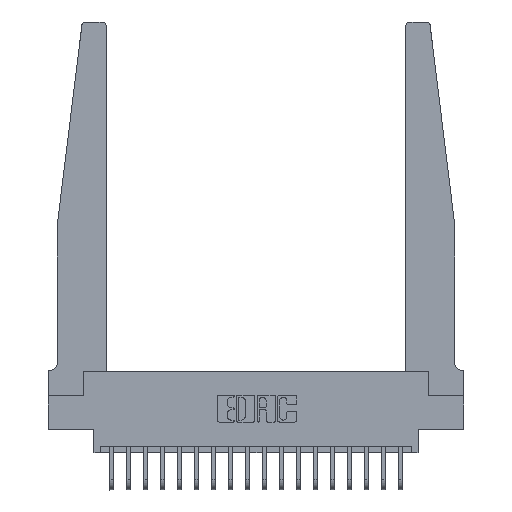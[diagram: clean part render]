
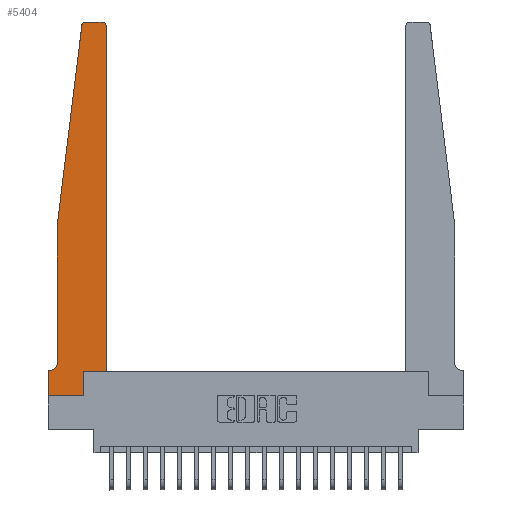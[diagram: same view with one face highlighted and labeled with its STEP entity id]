
A CAD part, top view. The second image highlights one B-rep face of the part: STEP entity #5404.
In plain terms, the highlighted planar face has unit normal (0, 0, 1).
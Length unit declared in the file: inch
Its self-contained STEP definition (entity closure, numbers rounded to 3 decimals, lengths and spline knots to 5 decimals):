
#7 = DIRECTION ( 'NONE',  ( 0., 0., -1. ) ) ;
#114 = DIRECTION ( 'NONE',  ( 1., 0., 0. ) ) ;
#468 = CARTESIAN_POINT ( 'NONE',  ( 0.24675, 2.72367, 0.37 ) ) ;
#535 = EDGE_CURVE ( 'NONE', #9507, #10295, #10881, .T. ) ;
#549 = VERTEX_POINT ( 'NONE', #468 ) ;
#550 = CIRCLE ( 'NONE', #14992, 0.03 ) ;
#697 = VERTEX_POINT ( 'NONE', #18527 ) ;
#717 = DIRECTION ( 'NONE',  ( 0., -1., 0. ) ) ;
#861 = DIRECTION ( 'NONE',  ( 0., 0., 1. ) ) ;
#1441 = CARTESIAN_POINT ( 'NONE',  ( 0., 0., 0.37 ) ) ;
#1549 = VECTOR ( 'NONE', #114, 39.37008 ) ;
#1551 = FACE_OUTER_BOUND ( 'NONE', #19303, .T. ) ;
#1722 = LINE ( 'NONE', #13590, #2767 ) ;
#2453 = CARTESIAN_POINT ( 'NONE',  ( 0.425, 0.18, 0.37 ) ) ;
#2677 = CARTESIAN_POINT ( 'NONE',  ( 0.2605, 0.18, 0.37 ) ) ;
#2767 = VECTOR ( 'NONE', #7425, 39.37008 ) ;
#2812 = VERTEX_POINT ( 'NONE', #18369 ) ;
#2819 = ORIENTED_EDGE ( 'NONE', *, *, #2838, .T. ) ;
#2838 = EDGE_CURVE ( 'NONE', #14471, #10114, #16302, .T. ) ;
#3021 = CARTESIAN_POINT ( 'NONE',  ( 0.065, 1.25, 0.37 ) ) ;
#3446 = DIRECTION ( 'NONE',  ( 0., 0., 1. ) ) ;
#3517 = ORIENTED_EDGE ( 'NONE', *, *, #6738, .T. ) ;
#3747 = CARTESIAN_POINT ( 'NONE',  ( 0.425, 0.18, 0.37 ) ) ;
#4168 = CARTESIAN_POINT ( 'NONE',  ( 0.425, 2.72, 0.37 ) ) ;
#4404 = ORIENTED_EDGE ( 'NONE', *, *, #9298, .T. ) ;
#5031 = DIRECTION ( 'NONE',  ( -1., 0., 0. ) ) ;
#5090 = CARTESIAN_POINT ( 'NONE',  ( 0.2605, 0., 0.37 ) ) ;
#5404 = ADVANCED_FACE ( 'NONE', ( #1551 ), #14762, .T. ) ;
#5718 = ORIENTED_EDGE ( 'NONE', *, *, #12366, .T. ) ;
#6118 = CIRCLE ( 'NONE', #12478, 0.03 ) ;
#6351 = EDGE_CURVE ( 'NONE', #10114, #13738, #1722, .T. ) ;
#6361 = DIRECTION ( 'NONE',  ( 1., 0., 0. ) ) ;
#6429 = EDGE_CURVE ( 'NONE', #12772, #21199, #9536, .T. ) ;
#6506 = CARTESIAN_POINT ( 'NONE',  ( 0., 0.1875, 0.37 ) ) ;
#6641 = LINE ( 'NONE', #11664, #10573 ) ;
#6738 = EDGE_CURVE ( 'NONE', #549, #10972, #9307, .T. ) ;
#6746 = ORIENTED_EDGE ( 'NONE', *, *, #6429, .T. ) ;
#6799 = VECTOR ( 'NONE', #16878, 39.37008 ) ;
#6945 = DIRECTION ( 'NONE',  ( -0.122, -0.992, 0. ) ) ;
#7122 = ORIENTED_EDGE ( 'NONE', *, *, #16498, .T. ) ;
#7391 = AXIS2_PLACEMENT_3D ( 'NONE', #20221, #7, #20282 ) ;
#7425 = DIRECTION ( 'NONE',  ( -1., 0., 0. ) ) ;
#7553 = DIRECTION ( 'NONE',  ( 0., 1., 0. ) ) ;
#7672 = EDGE_CURVE ( 'NONE', #10295, #2812, #6118, .T. ) ;
#7897 = EDGE_CURVE ( 'NONE', #2812, #697, #6641, .T. ) ;
#8036 = ORIENTED_EDGE ( 'NONE', *, *, #535, .T. ) ;
#9072 = CARTESIAN_POINT ( 'NONE',  ( 0., 0., 0.37 ) ) ;
#9298 = EDGE_CURVE ( 'NONE', #697, #549, #550, .T. ) ;
#9307 = LINE ( 'NONE', #17565, #16384 ) ;
#9326 = VECTOR ( 'NONE', #21129, 39.37008 ) ;
#9507 = VERTEX_POINT ( 'NONE', #3747 ) ;
#9510 = CARTESIAN_POINT ( 'NONE',  ( 0., 0.1875, 0.37 ) ) ;
#9536 = LINE ( 'NONE', #2677, #9326 ) ;
#9836 = VECTOR ( 'NONE', #16049, 39.37008 ) ;
#10013 = CARTESIAN_POINT ( 'NONE',  ( 0.2605, 0.18, 0.37 ) ) ;
#10114 = VERTEX_POINT ( 'NONE', #18724 ) ;
#10295 = VERTEX_POINT ( 'NONE', #4168 ) ;
#10573 = VECTOR ( 'NONE', #5031, 39.37008 ) ;
#10617 = VECTOR ( 'NONE', #7553, 39.37008 ) ;
#10620 = DIRECTION ( 'NONE',  ( 1., 0., 0. ) ) ;
#10634 = EDGE_CURVE ( 'NONE', #10870, #12772, #17252, .T. ) ;
#10870 = VERTEX_POINT ( 'NONE', #14080 ) ;
#10881 = LINE ( 'NONE', #16935, #10617 ) ;
#10972 = VERTEX_POINT ( 'NONE', #3021 ) ;
#11229 = LINE ( 'NONE', #18343, #6799 ) ;
#11637 = LINE ( 'NONE', #2453, #9836 ) ;
#11664 = CARTESIAN_POINT ( 'NONE',  ( 0.25, 2.75, 0.37 ) ) ;
#12366 = EDGE_CURVE ( 'NONE', #13738, #10870, #19293, .T. ) ;
#12478 = AXIS2_PLACEMENT_3D ( 'NONE', #13370, #3446, #10620 ) ;
#12591 = ORIENTED_EDGE ( 'NONE', *, *, #7672, .T. ) ;
#12772 = VERTEX_POINT ( 'NONE', #5090 ) ;
#12907 = ORIENTED_EDGE ( 'NONE', *, *, #7897, .T. ) ;
#13370 = CARTESIAN_POINT ( 'NONE',  ( 0.395, 2.72, 0.37 ) ) ;
#13590 = CARTESIAN_POINT ( 'NONE',  ( 0.065, 0.1875, 0.37 ) ) ;
#13738 = VERTEX_POINT ( 'NONE', #9510 ) ;
#14080 = CARTESIAN_POINT ( 'NONE',  ( 0., 0., 0.37 ) ) ;
#14471 = VERTEX_POINT ( 'NONE', #16854 ) ;
#14659 = EDGE_CURVE ( 'NONE', #10972, #14471, #11229, .T. ) ;
#14762 = PLANE ( 'NONE',  #21441 ) ;
#14992 = AXIS2_PLACEMENT_3D ( 'NONE', #20934, #861, #17620 ) ;
#15229 = ORIENTED_EDGE ( 'NONE', *, *, #14659, .T. ) ;
#16049 = DIRECTION ( 'NONE',  ( 1., 0., 0. ) ) ;
#16302 = CIRCLE ( 'NONE', #7391, 0.05 ) ;
#16326 = ORIENTED_EDGE ( 'NONE', *, *, #10634, .T. ) ;
#16384 = VECTOR ( 'NONE', #6945, 39.37008 ) ;
#16498 = EDGE_CURVE ( 'NONE', #21199, #9507, #11637, .T. ) ;
#16854 = CARTESIAN_POINT ( 'NONE',  ( 0.065, 0.2375, 0.37 ) ) ;
#16878 = DIRECTION ( 'NONE',  ( 0., -1., 0. ) ) ;
#16929 = VECTOR ( 'NONE', #717, 39.37008 ) ;
#16935 = CARTESIAN_POINT ( 'NONE',  ( 0.425, 0.18, 0.37 ) ) ;
#17252 = LINE ( 'NONE', #1441, #1549 ) ;
#17565 = CARTESIAN_POINT ( 'NONE',  ( 0.065, 1.25, 0.37 ) ) ;
#17620 = DIRECTION ( 'NONE',  ( 1., 0., 0. ) ) ;
#18279 = DIRECTION ( 'NONE',  ( 0., 0., 1. ) ) ;
#18343 = CARTESIAN_POINT ( 'NONE',  ( 0.065, 1.25, 0.37 ) ) ;
#18369 = CARTESIAN_POINT ( 'NONE',  ( 0.395, 2.75, 0.37 ) ) ;
#18527 = CARTESIAN_POINT ( 'NONE',  ( 0.27653, 2.75, 0.37 ) ) ;
#18724 = CARTESIAN_POINT ( 'NONE',  ( 0.015, 0.1875, 0.37 ) ) ;
#19293 = LINE ( 'NONE', #9072, #16929 ) ;
#19303 = EDGE_LOOP ( 'NONE', ( #12907, #4404, #3517, #15229, #2819, #19679, #5718, #16326, #6746, #7122, #8036, #12591 ) ) ;
#19679 = ORIENTED_EDGE ( 'NONE', *, *, #6351, .T. ) ;
#20221 = CARTESIAN_POINT ( 'NONE',  ( 0.015, 0.2375, 0.37 ) ) ;
#20282 = DIRECTION ( 'NONE',  ( -1., 0., 0. ) ) ;
#20934 = CARTESIAN_POINT ( 'NONE',  ( 0.27653, 2.72, 0.37 ) ) ;
#21129 = DIRECTION ( 'NONE',  ( 0., 1., 0. ) ) ;
#21199 = VERTEX_POINT ( 'NONE', #10013 ) ;
#21441 = AXIS2_PLACEMENT_3D ( 'NONE', #6506, #18279, #6361 ) ;
